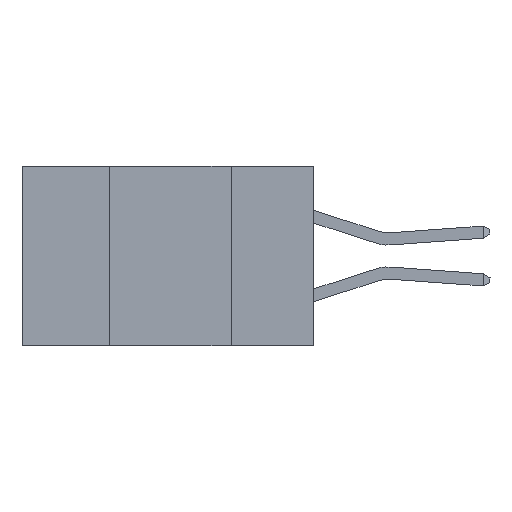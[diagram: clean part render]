
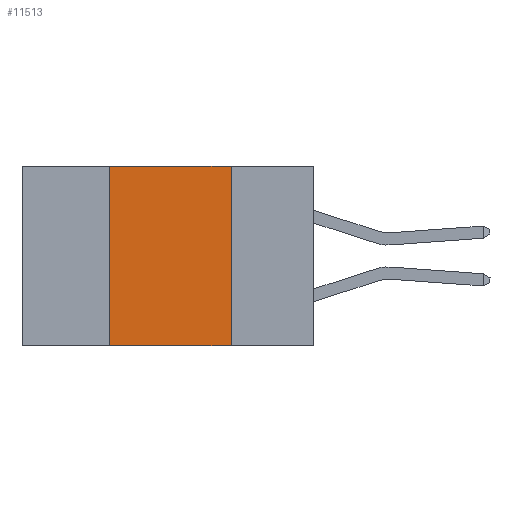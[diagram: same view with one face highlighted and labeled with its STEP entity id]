
A CAD part, left-side view. The second image highlights one B-rep face of the part: STEP entity #11513.
In plain terms, the highlighted planar face has unit normal (-1, 0, 0).
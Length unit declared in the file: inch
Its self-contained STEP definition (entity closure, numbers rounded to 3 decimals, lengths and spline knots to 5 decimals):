
#370 = LINE ( 'NONE', #30291, #15021 ) ;
#2164 = ORIENTED_EDGE ( 'NONE', *, *, #32880, .F. ) ;
#2671 = EDGE_CURVE ( 'NONE', #31091, #9559, #27812, .T. ) ;
#3871 = CARTESIAN_POINT ( 'NONE',  ( 0., 0.42, 0. ) ) ;
#4165 = CARTESIAN_POINT ( 'NONE',  ( 0., 0.42, 0. ) ) ;
#4418 = EDGE_LOOP ( 'NONE', ( #2164, #31293, #7841, #18407 ) ) ;
#5328 = CARTESIAN_POINT ( 'NONE',  ( 0., 0.42, -0.37 ) ) ;
#7190 = DIRECTION ( 'NONE',  ( 0., -1., 0. ) ) ;
#7841 = ORIENTED_EDGE ( 'NONE', *, *, #2671, .F. ) ;
#8465 = DIRECTION ( 'NONE',  ( 0., 0., 1. ) ) ;
#9559 = VERTEX_POINT ( 'NONE', #4165 ) ;
#10448 = EDGE_CURVE ( 'NONE', #31091, #10745, #29225, .T. ) ;
#10463 = DIRECTION ( 'NONE',  ( 0., -1., 0. ) ) ;
#10745 = VERTEX_POINT ( 'NONE', #22794 ) ;
#11089 = PLANE ( 'NONE',  #26838 ) ;
#11513 = ADVANCED_FACE ( 'NONE', ( #15988 ), #11089, .F. ) ;
#11689 = CARTESIAN_POINT ( 'NONE',  ( 0., 0.17, 0. ) ) ;
#12948 = CARTESIAN_POINT ( 'NONE',  ( 0., 0.6, -0.37 ) ) ;
#13691 = DIRECTION ( 'NONE',  ( 1., 0., 0. ) ) ;
#15021 = VECTOR ( 'NONE', #7190, 39.37008 ) ;
#15988 = FACE_OUTER_BOUND ( 'NONE', #4418, .T. ) ;
#17692 = CARTESIAN_POINT ( 'NONE',  ( 0., 0.17, 0. ) ) ;
#18008 = VECTOR ( 'NONE', #8465, 39.37008 ) ;
#18407 = ORIENTED_EDGE ( 'NONE', *, *, #10448, .T. ) ;
#19984 = DIRECTION ( 'NONE',  ( 0., 0., -1. ) ) ;
#21551 = DIRECTION ( 'NONE',  ( 0., 0., -1. ) ) ;
#22271 = VECTOR ( 'NONE', #10463, 39.37008 ) ;
#22794 = CARTESIAN_POINT ( 'NONE',  ( 0., 0.17, -0.37 ) ) ;
#24215 = VECTOR ( 'NONE', #19984, 39.37008 ) ;
#25728 = EDGE_CURVE ( 'NONE', #9559, #25897, #370, .T. ) ;
#25897 = VERTEX_POINT ( 'NONE', #11689 ) ;
#26838 = AXIS2_PLACEMENT_3D ( 'NONE', #31911, #13691, #21551 ) ;
#27812 = LINE ( 'NONE', #3871, #18008 ) ;
#29225 = LINE ( 'NONE', #12948, #22271 ) ;
#30291 = CARTESIAN_POINT ( 'NONE',  ( 0., 0.6, 0. ) ) ;
#31091 = VERTEX_POINT ( 'NONE', #5328 ) ;
#31147 = LINE ( 'NONE', #17692, #24215 ) ;
#31293 = ORIENTED_EDGE ( 'NONE', *, *, #25728, .F. ) ;
#31911 = CARTESIAN_POINT ( 'NONE',  ( 0., 0.6, 0. ) ) ;
#32880 = EDGE_CURVE ( 'NONE', #25897, #10745, #31147, .T. ) ;
